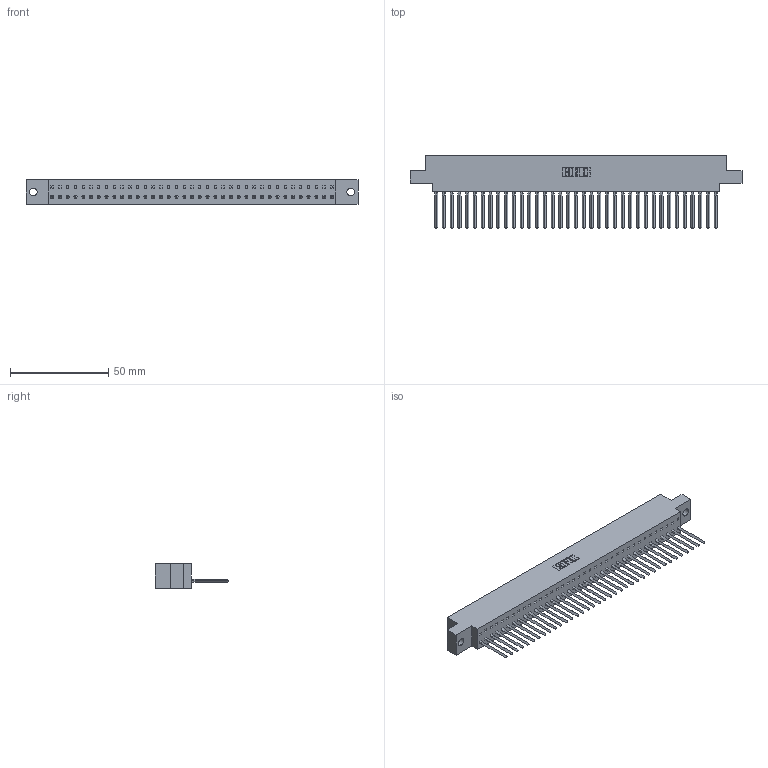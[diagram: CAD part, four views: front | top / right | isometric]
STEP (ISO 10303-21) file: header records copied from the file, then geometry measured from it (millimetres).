
FILE_DESCRIPTION (( 'STEP AP203' ), '1' );
FILE_NAME ('317-037-541-604.STEP', '2020-02-27T23:13:50', ( '' ), ( '' ), 'SwSTEP 2.0', 'SolidWorks 2016', '' );
FILE_SCHEMA (( 'CONFIG_CONTROL_DESIGN' ));
Length unit declared in the file: inch
Products named in the file (3): 317-290-002_541; 317 Part_.156 Dia - TH; 317-037-541-604
Assembly tree (38 placements, depth 2):
  317-037-541-604
    317 Part_.156 Dia - TH
    317-290-002_541  x37
Bounding box: 169.32 x 37.34 x 12.7 mm (x, y, z)
Volume: 27215.8 mm3; surface area: 38109.1 mm2
Topology: 38 solids, 38 shells, 5726 faces, 16333 edges, 10616 vertices
Faces by surface type: plane 4646, cylinder 932, bspline 148
Entity records: 54548 total; most frequent: CARTESIAN_POINT 10336, ORIENTED_EDGE 9626, DIRECTION 7903, EDGE_CURVE 4813, VECTOR 4449, LINE 4449, VERTEX_POINT 3200, AXIS2_PLACEMENT_3D 1727
